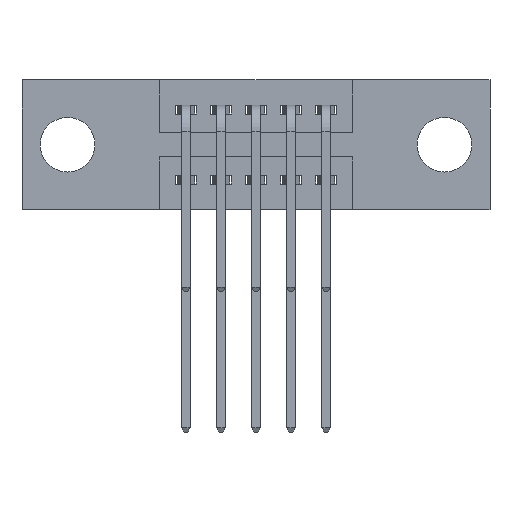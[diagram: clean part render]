
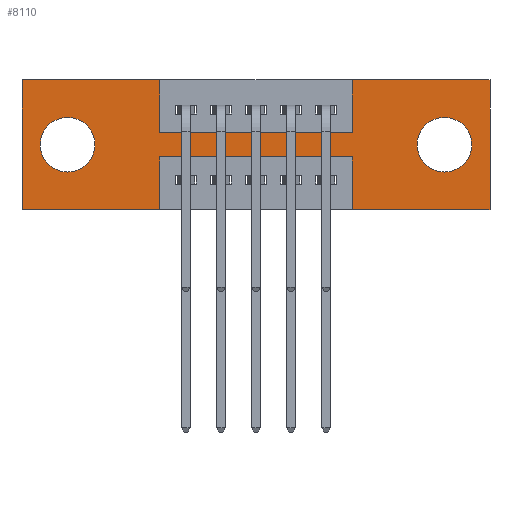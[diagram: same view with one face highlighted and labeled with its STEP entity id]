
A CAD part, front view. The second image highlights one B-rep face of the part: STEP entity #8110.
In plain terms, the highlighted planar face has unit normal (0, -1, 0).
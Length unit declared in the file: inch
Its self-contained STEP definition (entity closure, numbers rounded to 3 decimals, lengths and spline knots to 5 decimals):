
#15 = LINE ( 'NONE', #9555, #8075 ) ;
#118 = VERTEX_POINT ( 'NONE', #5343 ) ;
#345 = DIRECTION ( 'NONE',  ( 0., 1., 0. ) ) ;
#368 = ORIENTED_EDGE ( 'NONE', *, *, #10202, .F. ) ;
#468 = DIRECTION ( 'NONE',  ( 0., 0., 1. ) ) ;
#469 = CARTESIAN_POINT ( 'NONE',  ( 0.3925, 0., 0. ) ) ;
#580 = EDGE_CURVE ( 'NONE', #8156, #10264, #3062, .T. ) ;
#615 = EDGE_CURVE ( 'NONE', #5859, #6043, #5043, .T. ) ;
#713 = VERTEX_POINT ( 'NONE', #3242 ) ;
#1004 = DIRECTION ( 'NONE',  ( 0., 1., 0. ) ) ;
#1044 = VECTOR ( 'NONE', #10175, 39.37008 ) ;
#1199 = DIRECTION ( 'NONE',  ( 0., 0., 1. ) ) ;
#1272 = AXIS2_PLACEMENT_3D ( 'NONE', #10154, #1004, #3883 ) ;
#1315 = CARTESIAN_POINT ( 'NONE',  ( 0., 0., -0.37 ) ) ;
#1540 = AXIS2_PLACEMENT_3D ( 'NONE', #3170, #8954, #4018 ) ;
#1565 = ORIENTED_EDGE ( 'NONE', *, *, #9264, .F. ) ;
#1749 = AXIS2_PLACEMENT_3D ( 'NONE', #5344, #345, #6167 ) ;
#1759 = CARTESIAN_POINT ( 'NONE',  ( 0.9425, 0., 0. ) ) ;
#1804 = CARTESIAN_POINT ( 'NONE',  ( 0., 0., 0. ) ) ;
#1861 = CIRCLE ( 'NONE', #1540, 0.078 ) ;
#1929 = ORIENTED_EDGE ( 'NONE', *, *, #2558, .F. ) ;
#2163 = EDGE_CURVE ( 'NONE', #9398, #8140, #6427, .T. ) ;
#2200 = ORIENTED_EDGE ( 'NONE', *, *, #615, .F. ) ;
#2331 = ORIENTED_EDGE ( 'NONE', *, *, #3798, .F. ) ;
#2361 = EDGE_CURVE ( 'NONE', #6043, #5745, #4075, .T. ) ;
#2505 = CARTESIAN_POINT ( 'NONE',  ( 0., 0., 0. ) ) ;
#2558 = EDGE_CURVE ( 'NONE', #3554, #4053, #15, .T. ) ;
#2561 = CARTESIAN_POINT ( 'NONE',  ( 0., 0., -0.37 ) ) ;
#2592 = CARTESIAN_POINT ( 'NONE',  ( 1.335, 0., -0.37 ) ) ;
#2618 = EDGE_CURVE ( 'NONE', #713, #3554, #5658, .T. ) ;
#2691 = CARTESIAN_POINT ( 'NONE',  ( 0.9425, 0., 0. ) ) ;
#2794 = VECTOR ( 'NONE', #3756, 39.37008 ) ;
#2962 = ORIENTED_EDGE ( 'NONE', *, *, #2361, .F. ) ;
#3062 = CIRCLE ( 'NONE', #3899, 0.078 ) ;
#3072 = LINE ( 'NONE', #7798, #4805 ) ;
#3170 = CARTESIAN_POINT ( 'NONE',  ( 1.205, 0., -0.185 ) ) ;
#3242 = CARTESIAN_POINT ( 'NONE',  ( 0.3925, 0., -0.22 ) ) ;
#3331 = DIRECTION ( 'NONE',  ( 1., 0., 0. ) ) ;
#3363 = ORIENTED_EDGE ( 'NONE', *, *, #5147, .F. ) ;
#3397 = PLANE ( 'NONE',  #5434 ) ;
#3406 = CARTESIAN_POINT ( 'NONE',  ( 0.3925, 0., -0.37 ) ) ;
#3546 = VERTEX_POINT ( 'NONE', #469 ) ;
#3554 = VERTEX_POINT ( 'NONE', #3406 ) ;
#3660 = EDGE_CURVE ( 'NONE', #10264, #8156, #4857, .T. ) ;
#3720 = VECTOR ( 'NONE', #3808, 39.37008 ) ;
#3754 = ORIENTED_EDGE ( 'NONE', *, *, #2163, .F. ) ;
#3756 = DIRECTION ( 'NONE',  ( 1., 0., 0. ) ) ;
#3783 = LINE ( 'NONE', #9481, #1044 ) ;
#3798 = EDGE_CURVE ( 'NONE', #3546, #5859, #3783, .T. ) ;
#3808 = DIRECTION ( 'NONE',  ( -1., 0., 0. ) ) ;
#3840 = DIRECTION ( 'NONE',  ( -1., 0., 0. ) ) ;
#3883 = DIRECTION ( 'NONE',  ( 0., 0., 1. ) ) ;
#3899 = AXIS2_PLACEMENT_3D ( 'NONE', #4958, #10048, #468 ) ;
#3970 = FACE_BOUND ( 'NONE', #5786, .T. ) ;
#3987 = DIRECTION ( 'NONE',  ( 0., 0., -1. ) ) ;
#4012 = ORIENTED_EDGE ( 'NONE', *, *, #7251, .F. ) ;
#4018 = DIRECTION ( 'NONE',  ( 0., 0., -1. ) ) ;
#4023 = ORIENTED_EDGE ( 'NONE', *, *, #7162, .F. ) ;
#4042 = VERTEX_POINT ( 'NONE', #9635 ) ;
#4050 = VERTEX_POINT ( 'NONE', #9987 ) ;
#4053 = VERTEX_POINT ( 'NONE', #9497 ) ;
#4075 = LINE ( 'NONE', #2691, #10028 ) ;
#4175 = VERTEX_POINT ( 'NONE', #8157 ) ;
#4292 = EDGE_LOOP ( 'NONE', ( #8908, #8648 ) ) ;
#4697 = ORIENTED_EDGE ( 'NONE', *, *, #7354, .F. ) ;
#4805 = VECTOR ( 'NONE', #6181, 39.37008 ) ;
#4857 = CIRCLE ( 'NONE', #1272, 0.078 ) ;
#4914 = CARTESIAN_POINT ( 'NONE',  ( 0.3925, 0., -0.15 ) ) ;
#4958 = CARTESIAN_POINT ( 'NONE',  ( 0.13, 0., -0.185 ) ) ;
#5001 = CIRCLE ( 'NONE', #1749, 0.078 ) ;
#5043 = LINE ( 'NONE', #4914, #2794 ) ;
#5120 = CARTESIAN_POINT ( 'NONE',  ( 0.13, 0., -0.263 ) ) ;
#5127 = CARTESIAN_POINT ( 'NONE',  ( 0., 0., 0. ) ) ;
#5147 = EDGE_CURVE ( 'NONE', #5745, #9398, #5984, .T. ) ;
#5192 = CARTESIAN_POINT ( 'NONE',  ( 0.9425, 0., -0.22 ) ) ;
#5343 = CARTESIAN_POINT ( 'NONE',  ( 0.9425, 0., -0.37 ) ) ;
#5344 = CARTESIAN_POINT ( 'NONE',  ( 1.205, 0., -0.185 ) ) ;
#5434 = AXIS2_PLACEMENT_3D ( 'NONE', #2561, #9884, #9162 ) ;
#5658 = LINE ( 'NONE', #6038, #7566 ) ;
#5726 = ORIENTED_EDGE ( 'NONE', *, *, #2618, .F. ) ;
#5745 = VERTEX_POINT ( 'NONE', #1759 ) ;
#5786 = EDGE_LOOP ( 'NONE', ( #7768, #6349 ) ) ;
#5859 = VERTEX_POINT ( 'NONE', #9269 ) ;
#5864 = VERTEX_POINT ( 'NONE', #5192 ) ;
#5937 = DIRECTION ( 'NONE',  ( 0., 0., -1. ) ) ;
#5966 = LINE ( 'NONE', #1315, #3720 ) ;
#5984 = LINE ( 'NONE', #1804, #7884 ) ;
#6038 = CARTESIAN_POINT ( 'NONE',  ( 0.3925, 0., -0.37 ) ) ;
#6043 = VERTEX_POINT ( 'NONE', #10206 ) ;
#6066 = CARTESIAN_POINT ( 'NONE',  ( 0.13, 0., -0.107 ) ) ;
#6167 = DIRECTION ( 'NONE',  ( 0., 0., -1. ) ) ;
#6181 = DIRECTION ( 'NONE',  ( 0., 0., 1. ) ) ;
#6182 = FACE_BOUND ( 'NONE', #4292, .T. ) ;
#6349 = ORIENTED_EDGE ( 'NONE', *, *, #580, .T. ) ;
#6427 = LINE ( 'NONE', #7432, #8588 ) ;
#6826 = VECTOR ( 'NONE', #3331, 39.37008 ) ;
#7111 = VECTOR ( 'NONE', #10416, 39.37008 ) ;
#7162 = EDGE_CURVE ( 'NONE', #118, #5864, #3072, .T. ) ;
#7251 = EDGE_CURVE ( 'NONE', #8140, #118, #5966, .T. ) ;
#7354 = EDGE_CURVE ( 'NONE', #5864, #713, #9736, .T. ) ;
#7432 = CARTESIAN_POINT ( 'NONE',  ( 1.335, 0., 0. ) ) ;
#7566 = VECTOR ( 'NONE', #5937, 39.37008 ) ;
#7616 = DIRECTION ( 'NONE',  ( 1., 0., 0. ) ) ;
#7768 = ORIENTED_EDGE ( 'NONE', *, *, #3660, .T. ) ;
#7798 = CARTESIAN_POINT ( 'NONE',  ( 0.9425, 0., -0.37 ) ) ;
#7884 = VECTOR ( 'NONE', #7616, 39.37008 ) ;
#7945 = LINE ( 'NONE', #5127, #10023 ) ;
#8075 = VECTOR ( 'NONE', #3840, 39.37008 ) ;
#8110 = ADVANCED_FACE ( 'NONE', ( #6182, #3970, #10169 ), #3397, .T. ) ;
#8140 = VERTEX_POINT ( 'NONE', #2592 ) ;
#8156 = VERTEX_POINT ( 'NONE', #5120 ) ;
#8157 = CARTESIAN_POINT ( 'NONE',  ( 0., 0., 0. ) ) ;
#8484 = CARTESIAN_POINT ( 'NONE',  ( 1.335, 0., 0. ) ) ;
#8588 = VECTOR ( 'NONE', #3987, 39.37008 ) ;
#8648 = ORIENTED_EDGE ( 'NONE', *, *, #10334, .T. ) ;
#8785 = EDGE_LOOP ( 'NONE', ( #5726, #4697, #4023, #4012, #3754, #3363, #2962, #2200, #2331, #1565, #368, #1929 ) ) ;
#8908 = ORIENTED_EDGE ( 'NONE', *, *, #9641, .T. ) ;
#8954 = DIRECTION ( 'NONE',  ( 0., 1., 0. ) ) ;
#9162 = DIRECTION ( 'NONE',  ( 0., 0., -1. ) ) ;
#9236 = LINE ( 'NONE', #2505, #6826 ) ;
#9264 = EDGE_CURVE ( 'NONE', #4175, #3546, #9236, .T. ) ;
#9269 = CARTESIAN_POINT ( 'NONE',  ( 0.3925, 0., -0.15 ) ) ;
#9398 = VERTEX_POINT ( 'NONE', #8484 ) ;
#9481 = CARTESIAN_POINT ( 'NONE',  ( 0.3925, 0., 0. ) ) ;
#9497 = CARTESIAN_POINT ( 'NONE',  ( 0., 0., -0.37 ) ) ;
#9555 = CARTESIAN_POINT ( 'NONE',  ( 0., 0., -0.37 ) ) ;
#9635 = CARTESIAN_POINT ( 'NONE',  ( 1.205, 0., -0.263 ) ) ;
#9641 = EDGE_CURVE ( 'NONE', #4050, #4042, #1861, .T. ) ;
#9674 = CARTESIAN_POINT ( 'NONE',  ( 0.3925, 0., -0.22 ) ) ;
#9736 = LINE ( 'NONE', #9674, #7111 ) ;
#9884 = DIRECTION ( 'NONE',  ( 0., -1., 0. ) ) ;
#9952 = DIRECTION ( 'NONE',  ( 0., 0., 1. ) ) ;
#9987 = CARTESIAN_POINT ( 'NONE',  ( 1.205, 0., -0.107 ) ) ;
#10023 = VECTOR ( 'NONE', #9952, 39.37008 ) ;
#10028 = VECTOR ( 'NONE', #1199, 39.37008 ) ;
#10048 = DIRECTION ( 'NONE',  ( 0., 1., 0. ) ) ;
#10154 = CARTESIAN_POINT ( 'NONE',  ( 0.13, 0., -0.185 ) ) ;
#10169 = FACE_OUTER_BOUND ( 'NONE', #8785, .T. ) ;
#10175 = DIRECTION ( 'NONE',  ( 0., 0., -1. ) ) ;
#10202 = EDGE_CURVE ( 'NONE', #4053, #4175, #7945, .T. ) ;
#10206 = CARTESIAN_POINT ( 'NONE',  ( 0.9425, 0., -0.15 ) ) ;
#10264 = VERTEX_POINT ( 'NONE', #6066 ) ;
#10334 = EDGE_CURVE ( 'NONE', #4042, #4050, #5001, .T. ) ;
#10416 = DIRECTION ( 'NONE',  ( -1., 0., 0. ) ) ;
